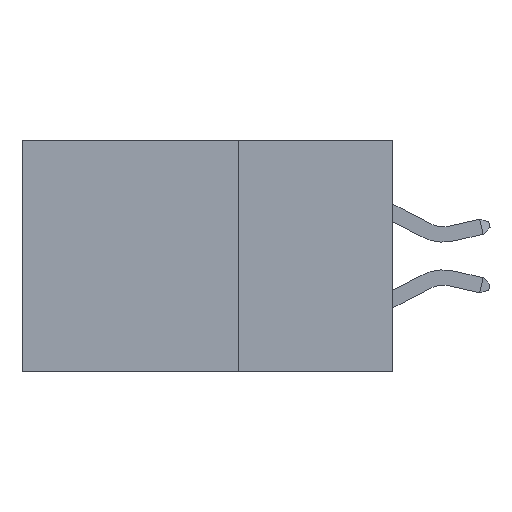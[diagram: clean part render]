
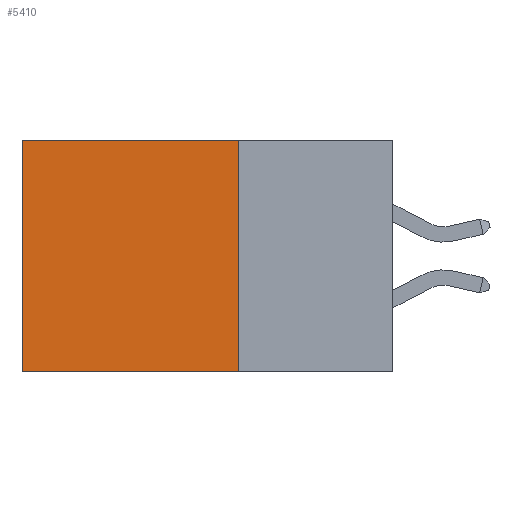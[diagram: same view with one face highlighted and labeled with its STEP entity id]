
A CAD part, left-side view. The second image highlights one B-rep face of the part: STEP entity #5410.
In plain terms, the highlighted planar face has unit normal (-1, 0, 0).
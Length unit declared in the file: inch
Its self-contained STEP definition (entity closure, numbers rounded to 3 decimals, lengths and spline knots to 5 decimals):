
#175 = ORIENTED_EDGE ( 'NONE', *, *, #5844, .T. ) ;
#1051 = VECTOR ( 'NONE', #5787, 39.37008 ) ;
#1072 = CARTESIAN_POINT ( 'NONE',  ( 0.2875, 0.6, -0.375 ) ) ;
#2508 = VECTOR ( 'NONE', #6709, 39.37008 ) ;
#3709 = LINE ( 'NONE', #10210, #6938 ) ;
#3797 = EDGE_CURVE ( 'NONE', #13813, #4909, #6568, .T. ) ;
#4543 = CARTESIAN_POINT ( 'NONE',  ( 0.2875, 0.25, 0. ) ) ;
#4638 = DIRECTION ( 'NONE',  ( 0., 0., -1. ) ) ;
#4909 = VERTEX_POINT ( 'NONE', #10030 ) ;
#5410 = ADVANCED_FACE ( 'NONE', ( #8816 ), #11219, .F. ) ;
#5787 = DIRECTION ( 'NONE',  ( 0., 0., -1. ) ) ;
#5844 = EDGE_CURVE ( 'NONE', #13813, #7169, #3709, .T. ) ;
#6568 = LINE ( 'NONE', #10029, #2508 ) ;
#6709 = DIRECTION ( 'NONE',  ( 0., 0., -1. ) ) ;
#6838 = ORIENTED_EDGE ( 'NONE', *, *, #3797, .F. ) ;
#6938 = VECTOR ( 'NONE', #12249, 39.37008 ) ;
#7169 = VERTEX_POINT ( 'NONE', #11342 ) ;
#7448 = ORIENTED_EDGE ( 'NONE', *, *, #12927, .T. ) ;
#7495 = EDGE_CURVE ( 'NONE', #4909, #13224, #12236, .T. ) ;
#7799 = EDGE_LOOP ( 'NONE', ( #7448, #8314, #6838, #175 ) ) ;
#7937 = DIRECTION ( 'NONE',  ( 0., 1., 0. ) ) ;
#8314 = ORIENTED_EDGE ( 'NONE', *, *, #7495, .F. ) ;
#8816 = FACE_OUTER_BOUND ( 'NONE', #7799, .T. ) ;
#9774 = CARTESIAN_POINT ( 'NONE',  ( 0.2875, 0.25, -0.375 ) ) ;
#9909 = VECTOR ( 'NONE', #7937, 39.37008 ) ;
#10029 = CARTESIAN_POINT ( 'NONE',  ( 0.2875, 0.25, -0.375 ) ) ;
#10030 = CARTESIAN_POINT ( 'NONE',  ( 0.2875, 0.25, -0.375 ) ) ;
#10115 = AXIS2_PLACEMENT_3D ( 'NONE', #13110, #11007, #4638 ) ;
#10210 = CARTESIAN_POINT ( 'NONE',  ( 0.2875, 0.25, 0. ) ) ;
#10957 = CARTESIAN_POINT ( 'NONE',  ( 0.2875, 0.6, -0.375 ) ) ;
#11007 = DIRECTION ( 'NONE',  ( 1., 0., 0. ) ) ;
#11219 = PLANE ( 'NONE',  #10115 ) ;
#11342 = CARTESIAN_POINT ( 'NONE',  ( 0.2875, 0.6, 0. ) ) ;
#12012 = LINE ( 'NONE', #10957, #1051 ) ;
#12236 = LINE ( 'NONE', #9774, #9909 ) ;
#12249 = DIRECTION ( 'NONE',  ( 0., 1., 0. ) ) ;
#12927 = EDGE_CURVE ( 'NONE', #7169, #13224, #12012, .T. ) ;
#13110 = CARTESIAN_POINT ( 'NONE',  ( 0.2875, 0.25, -0.375 ) ) ;
#13224 = VERTEX_POINT ( 'NONE', #1072 ) ;
#13813 = VERTEX_POINT ( 'NONE', #4543 ) ;
